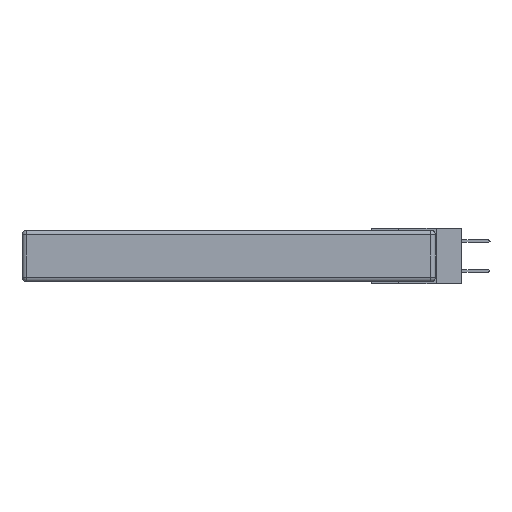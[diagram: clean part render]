
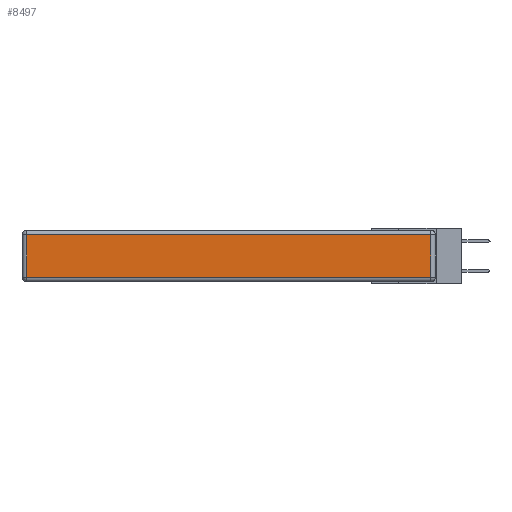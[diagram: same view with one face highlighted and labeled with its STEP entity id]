
A CAD part, left-side view. The second image highlights one B-rep face of the part: STEP entity #8497.
In plain terms, the highlighted planar face has unit normal (-1, 0, 0).
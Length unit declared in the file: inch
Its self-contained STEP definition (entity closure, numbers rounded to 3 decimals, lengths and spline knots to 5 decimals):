
#1507 = VERTEX_POINT ( 'NONE', #15052 ) ;
#2389 = PLANE ( 'NONE',  #12637 ) ;
#2938 = LINE ( 'NONE', #21015, #22898 ) ;
#3530 = DIRECTION ( 'NONE',  ( 0., -1., 0. ) ) ;
#4875 = EDGE_LOOP ( 'NONE', ( #18098, #8562, #31348, #31186 ) ) ;
#5183 = EDGE_CURVE ( 'NONE', #1507, #21189, #20614, .T. ) ;
#5398 = LINE ( 'NONE', #23409, #30777 ) ;
#6175 = DIRECTION ( 'NONE',  ( 0., 0., -1. ) ) ;
#7733 = CARTESIAN_POINT ( 'NONE',  ( 0., 2.72, -0.343 ) ) ;
#7878 = DIRECTION ( 'NONE',  ( 0., 0., 1. ) ) ;
#8497 = ADVANCED_FACE ( 'NONE', ( #18783 ), #2389, .T. ) ;
#8506 = VECTOR ( 'NONE', #21883, 39.37008 ) ;
#8562 = ORIENTED_EDGE ( 'NONE', *, *, #23015, .T. ) ;
#11070 = EDGE_CURVE ( 'NONE', #21263, #29787, #2938, .T. ) ;
#11078 = DIRECTION ( 'NONE',  ( 0., 0., 1. ) ) ;
#12637 = AXIS2_PLACEMENT_3D ( 'NONE', #25321, #22423, #7878 ) ;
#15052 = CARTESIAN_POINT ( 'NONE',  ( 0., 0.03, -0.03 ) ) ;
#18098 = ORIENTED_EDGE ( 'NONE', *, *, #11070, .T. ) ;
#18783 = FACE_OUTER_BOUND ( 'NONE', #4875, .T. ) ;
#18858 = VECTOR ( 'NONE', #6175, 39.37008 ) ;
#19651 = LINE ( 'NONE', #7733, #18858 ) ;
#20293 = EDGE_CURVE ( 'NONE', #21189, #21263, #19651, .T. ) ;
#20614 = LINE ( 'NONE', #24602, #8506 ) ;
#21015 = CARTESIAN_POINT ( 'NONE',  ( 0., 0., -0.313 ) ) ;
#21189 = VERTEX_POINT ( 'NONE', #26384 ) ;
#21263 = VERTEX_POINT ( 'NONE', #25950 ) ;
#21883 = DIRECTION ( 'NONE',  ( 0., 1., 0. ) ) ;
#22423 = DIRECTION ( 'NONE',  ( -1., 0., 0. ) ) ;
#22898 = VECTOR ( 'NONE', #3530, 39.37008 ) ;
#23015 = EDGE_CURVE ( 'NONE', #29787, #1507, #5398, .T. ) ;
#23409 = CARTESIAN_POINT ( 'NONE',  ( 0., 0.03, -0.343 ) ) ;
#24602 = CARTESIAN_POINT ( 'NONE',  ( 0., 2.75, -0.03 ) ) ;
#25321 = CARTESIAN_POINT ( 'NONE',  ( 0., 0., -0.343 ) ) ;
#25702 = CARTESIAN_POINT ( 'NONE',  ( 0., 0.03, -0.313 ) ) ;
#25950 = CARTESIAN_POINT ( 'NONE',  ( 0., 2.72, -0.313 ) ) ;
#26384 = CARTESIAN_POINT ( 'NONE',  ( 0., 2.72, -0.03 ) ) ;
#29787 = VERTEX_POINT ( 'NONE', #25702 ) ;
#30777 = VECTOR ( 'NONE', #11078, 39.37008 ) ;
#31186 = ORIENTED_EDGE ( 'NONE', *, *, #20293, .T. ) ;
#31348 = ORIENTED_EDGE ( 'NONE', *, *, #5183, .T. ) ;
